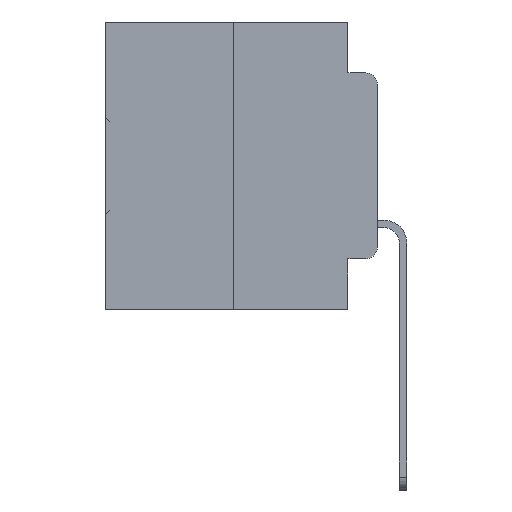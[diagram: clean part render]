
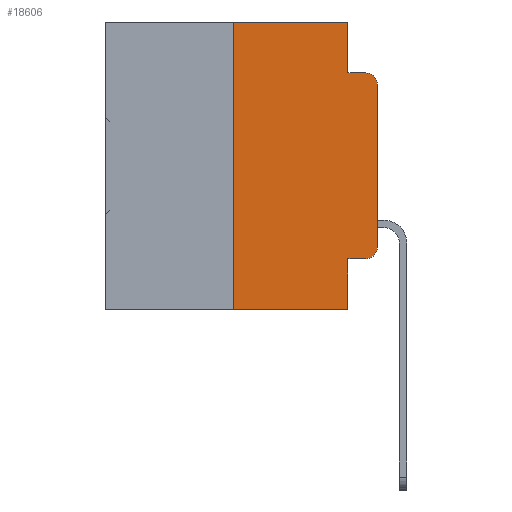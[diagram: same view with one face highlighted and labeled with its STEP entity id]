
A CAD part, left-side view. The second image highlights one B-rep face of the part: STEP entity #18606.
In plain terms, the highlighted planar face has unit normal (-1, 0, 0).
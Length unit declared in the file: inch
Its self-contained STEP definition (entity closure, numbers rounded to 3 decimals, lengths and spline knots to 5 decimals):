
#666 = ORIENTED_EDGE ( 'NONE', *, *, #5639, .F. ) ;
#1149 = EDGE_CURVE ( 'NONE', #23413, #19639, #9950, .T. ) ;
#1210 = ORIENTED_EDGE ( 'NONE', *, *, #14485, .T. ) ;
#3050 = VERTEX_POINT ( 'NONE', #23437 ) ;
#3138 = LINE ( 'NONE', #15315, #31552 ) ;
#3456 = CARTESIAN_POINT ( 'NONE',  ( 0., 0.473, 0. ) ) ;
#4655 = CARTESIAN_POINT ( 'NONE',  ( 0., 0.051, -0.0885 ) ) ;
#5028 = VECTOR ( 'NONE', #35417, 39.37008 ) ;
#5117 = LINE ( 'NONE', #11083, #25387 ) ;
#5639 = EDGE_CURVE ( 'NONE', #22697, #20684, #20568, .T. ) ;
#5731 = CARTESIAN_POINT ( 'NONE',  ( 0., 0.051, -0.0885 ) ) ;
#6270 = DIRECTION ( 'NONE',  ( 0., -1., 0. ) ) ;
#6404 = ORIENTED_EDGE ( 'NONE', *, *, #12649, .F. ) ;
#6646 = DIRECTION ( 'NONE',  ( -1., 0., 0. ) ) ;
#8119 = CIRCLE ( 'NONE', #31011, 0.02 ) ;
#8648 = DIRECTION ( 'NONE',  ( 0., 0., -1. ) ) ;
#8676 = CARTESIAN_POINT ( 'NONE',  ( 0., 0.02, -0.4115 ) ) ;
#9407 = VERTEX_POINT ( 'NONE', #33720 ) ;
#9491 = ORIENTED_EDGE ( 'NONE', *, *, #18500, .F. ) ;
#9662 = EDGE_LOOP ( 'NONE', ( #1210, #19167, #666, #9491, #6404, #33412, #30856, #30367, #30124, #10206 ) ) ;
#9919 = CARTESIAN_POINT ( 'NONE',  ( 0., 0.051, 0. ) ) ;
#9950 = LINE ( 'NONE', #24083, #23724 ) ;
#10206 = ORIENTED_EDGE ( 'NONE', *, *, #29157, .T. ) ;
#10520 = DIRECTION ( 'NONE',  ( 0., -1., 0. ) ) ;
#11083 = CARTESIAN_POINT ( 'NONE',  ( 0., 0.25, 0. ) ) ;
#11871 = DIRECTION ( 'NONE',  ( -1., 0., 0. ) ) ;
#12201 = CIRCLE ( 'NONE', #27221, 0.02 ) ;
#12649 = EDGE_CURVE ( 'NONE', #13626, #29329, #14587, .T. ) ;
#13626 = VERTEX_POINT ( 'NONE', #16773 ) ;
#14112 = CARTESIAN_POINT ( 'NONE',  ( 0., 0.473, 0. ) ) ;
#14485 = EDGE_CURVE ( 'NONE', #9407, #24372, #3138, .T. ) ;
#14587 = LINE ( 'NONE', #3456, #21050 ) ;
#15315 = CARTESIAN_POINT ( 'NONE',  ( 0., 0., 0. ) ) ;
#15362 = CARTESIAN_POINT ( 'NONE',  ( 0., 0.051, 0. ) ) ;
#16237 = CARTESIAN_POINT ( 'NONE',  ( 0., 0.25, -0.5 ) ) ;
#16773 = CARTESIAN_POINT ( 'NONE',  ( 0., 0.25, 0. ) ) ;
#18500 = EDGE_CURVE ( 'NONE', #29329, #22697, #34185, .T. ) ;
#18550 = LINE ( 'NONE', #15362, #32127 ) ;
#18606 = ADVANCED_FACE ( 'NONE', ( #32528 ), #33151, .F. ) ;
#18699 = EDGE_CURVE ( 'NONE', #24372, #20684, #8119, .T. ) ;
#18978 = EDGE_CURVE ( 'NONE', #3050, #19639, #18550, .T. ) ;
#19167 = ORIENTED_EDGE ( 'NONE', *, *, #18699, .T. ) ;
#19639 = VERTEX_POINT ( 'NONE', #23592 ) ;
#20360 = CARTESIAN_POINT ( 'NONE',  ( 0., 0.051, -0.4115 ) ) ;
#20568 = LINE ( 'NONE', #4655, #27783 ) ;
#20684 = VERTEX_POINT ( 'NONE', #21565 ) ;
#21050 = VECTOR ( 'NONE', #6270, 39.37008 ) ;
#21565 = CARTESIAN_POINT ( 'NONE',  ( 0., 0.02, -0.0885 ) ) ;
#22143 = DIRECTION ( 'NONE',  ( 0., 0., 1. ) ) ;
#22697 = VERTEX_POINT ( 'NONE', #5731 ) ;
#23212 = CARTESIAN_POINT ( 'NONE',  ( 0., 0.02, -0.1085 ) ) ;
#23413 = VERTEX_POINT ( 'NONE', #16237 ) ;
#23437 = CARTESIAN_POINT ( 'NONE',  ( 0., 0.051, -0.4115 ) ) ;
#23592 = CARTESIAN_POINT ( 'NONE',  ( 0., 0.051, -0.5 ) ) ;
#23724 = VECTOR ( 'NONE', #10520, 39.37008 ) ;
#23991 = DIRECTION ( 'NONE',  ( 0., -1., 0. ) ) ;
#24083 = CARTESIAN_POINT ( 'NONE',  ( 0., 0.473, -0.5 ) ) ;
#24372 = VERTEX_POINT ( 'NONE', #31744 ) ;
#24549 = CARTESIAN_POINT ( 'NONE',  ( 0., 0.051, 0. ) ) ;
#25110 = DIRECTION ( 'NONE',  ( 1., 0., 0. ) ) ;
#25387 = VECTOR ( 'NONE', #22143, 39.37008 ) ;
#25938 = DIRECTION ( 'NONE',  ( 0., 0., -1. ) ) ;
#26794 = VECTOR ( 'NONE', #31267, 39.37008 ) ;
#26912 = EDGE_CURVE ( 'NONE', #23413, #13626, #5117, .T. ) ;
#27221 = AXIS2_PLACEMENT_3D ( 'NONE', #28223, #11871, #30949 ) ;
#27616 = LINE ( 'NONE', #20360, #26794 ) ;
#27783 = VECTOR ( 'NONE', #23991, 39.37008 ) ;
#28223 = CARTESIAN_POINT ( 'NONE',  ( 0., 0.02, -0.3915 ) ) ;
#29157 = EDGE_CURVE ( 'NONE', #31443, #9407, #12201, .T. ) ;
#29329 = VERTEX_POINT ( 'NONE', #9919 ) ;
#29843 = EDGE_CURVE ( 'NONE', #3050, #31443, #27616, .T. ) ;
#30124 = ORIENTED_EDGE ( 'NONE', *, *, #29843, .T. ) ;
#30367 = ORIENTED_EDGE ( 'NONE', *, *, #18978, .F. ) ;
#30856 = ORIENTED_EDGE ( 'NONE', *, *, #1149, .T. ) ;
#30949 = DIRECTION ( 'NONE',  ( 0., 0., -1. ) ) ;
#31011 = AXIS2_PLACEMENT_3D ( 'NONE', #23212, #6646, #25938 ) ;
#31267 = DIRECTION ( 'NONE',  ( 0., -1., 0. ) ) ;
#31443 = VERTEX_POINT ( 'NONE', #8676 ) ;
#31552 = VECTOR ( 'NONE', #31631, 39.37008 ) ;
#31631 = DIRECTION ( 'NONE',  ( 0., 0., 1. ) ) ;
#31744 = CARTESIAN_POINT ( 'NONE',  ( 0., 0., -0.1085 ) ) ;
#32127 = VECTOR ( 'NONE', #34375, 39.37008 ) ;
#32528 = FACE_OUTER_BOUND ( 'NONE', #9662, .T. ) ;
#32861 = AXIS2_PLACEMENT_3D ( 'NONE', #14112, #25110, #8648 ) ;
#33151 = PLANE ( 'NONE',  #32861 ) ;
#33412 = ORIENTED_EDGE ( 'NONE', *, *, #26912, .F. ) ;
#33720 = CARTESIAN_POINT ( 'NONE',  ( 0., 0., -0.3915 ) ) ;
#34185 = LINE ( 'NONE', #24549, #5028 ) ;
#34375 = DIRECTION ( 'NONE',  ( 0., 0., -1. ) ) ;
#35417 = DIRECTION ( 'NONE',  ( 0., 0., -1. ) ) ;
